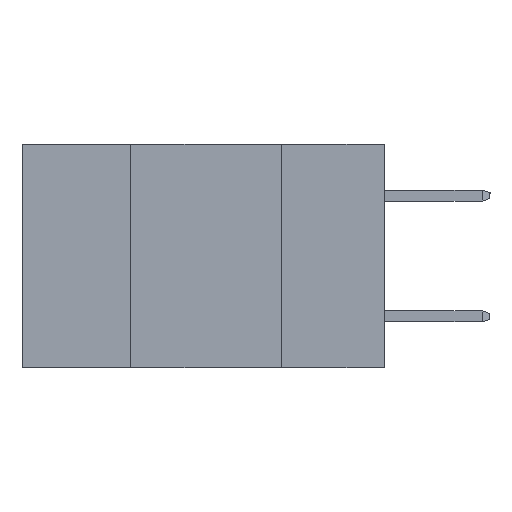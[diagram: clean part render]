
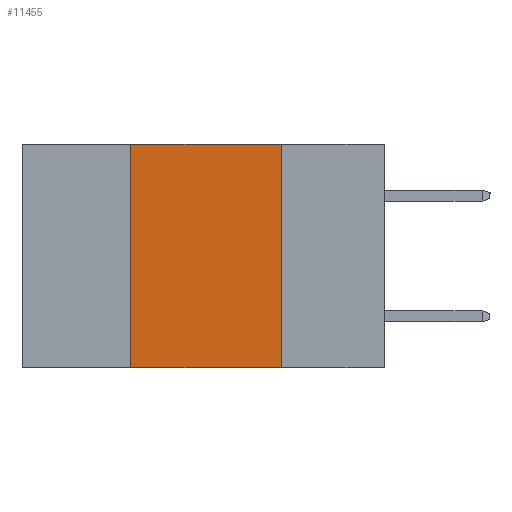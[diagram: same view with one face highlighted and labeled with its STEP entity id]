
A CAD part, left-side view. The second image highlights one B-rep face of the part: STEP entity #11455.
In plain terms, the highlighted planar face has unit normal (-1, 0, 0).
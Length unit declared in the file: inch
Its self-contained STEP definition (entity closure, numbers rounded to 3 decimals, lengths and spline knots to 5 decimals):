
#646 = DIRECTION ( 'NONE',  ( 1., 0., 0. ) ) ;
#749 = CARTESIAN_POINT ( 'NONE',  ( 0., 0.6, 0. ) ) ;
#812 = VECTOR ( 'NONE', #10671, 39.37008 ) ;
#945 = DIRECTION ( 'NONE',  ( 0., -1., 0. ) ) ;
#1645 = LINE ( 'NONE', #1781, #10247 ) ;
#1739 = VECTOR ( 'NONE', #3461, 39.37008 ) ;
#1781 = CARTESIAN_POINT ( 'NONE',  ( 0., 0.6, -0.37 ) ) ;
#1990 = ORIENTED_EDGE ( 'NONE', *, *, #8504, .T. ) ;
#2748 = FACE_OUTER_BOUND ( 'NONE', #5359, .T. ) ;
#3461 = DIRECTION ( 'NONE',  ( 0., 0., 1. ) ) ;
#3677 = VERTEX_POINT ( 'NONE', #7389 ) ;
#3715 = ORIENTED_EDGE ( 'NONE', *, *, #12449, .F. ) ;
#4160 = VERTEX_POINT ( 'NONE', #9693 ) ;
#4179 = EDGE_CURVE ( 'NONE', #4160, #9762, #10540, .T. ) ;
#5359 = EDGE_LOOP ( 'NONE', ( #6140, #3715, #9134, #1990 ) ) ;
#5480 = AXIS2_PLACEMENT_3D ( 'NONE', #6458, #646, #10487 ) ;
#6140 = ORIENTED_EDGE ( 'NONE', *, *, #4179, .F. ) ;
#6458 = CARTESIAN_POINT ( 'NONE',  ( 0., 0.6, 0. ) ) ;
#7389 = CARTESIAN_POINT ( 'NONE',  ( 0., 0.42, -0.37 ) ) ;
#7484 = CARTESIAN_POINT ( 'NONE',  ( 0., 0.42, -0.37 ) ) ;
#7616 = PLANE ( 'NONE',  #5480 ) ;
#8448 = VERTEX_POINT ( 'NONE', #12442 ) ;
#8504 = EDGE_CURVE ( 'NONE', #3677, #9762, #1645, .T. ) ;
#8795 = CARTESIAN_POINT ( 'NONE',  ( 0., 0.17, -0.37 ) ) ;
#8941 = EDGE_CURVE ( 'NONE', #3677, #8448, #12369, .T. ) ;
#9134 = ORIENTED_EDGE ( 'NONE', *, *, #8941, .F. ) ;
#9586 = DIRECTION ( 'NONE',  ( 0., -1., 0. ) ) ;
#9670 = VECTOR ( 'NONE', #945, 39.37008 ) ;
#9693 = CARTESIAN_POINT ( 'NONE',  ( 0., 0.17, 0. ) ) ;
#9762 = VERTEX_POINT ( 'NONE', #8795 ) ;
#10247 = VECTOR ( 'NONE', #9586, 39.37008 ) ;
#10487 = DIRECTION ( 'NONE',  ( 0., 0., -1. ) ) ;
#10540 = LINE ( 'NONE', #11717, #812 ) ;
#10671 = DIRECTION ( 'NONE',  ( 0., 0., -1. ) ) ;
#11455 = ADVANCED_FACE ( 'NONE', ( #2748 ), #7616, .F. ) ;
#11717 = CARTESIAN_POINT ( 'NONE',  ( 0., 0.17, -0.37 ) ) ;
#11759 = LINE ( 'NONE', #749, #9670 ) ;
#12369 = LINE ( 'NONE', #7484, #1739 ) ;
#12442 = CARTESIAN_POINT ( 'NONE',  ( 0., 0.42, 0. ) ) ;
#12449 = EDGE_CURVE ( 'NONE', #8448, #4160, #11759, .T. ) ;
